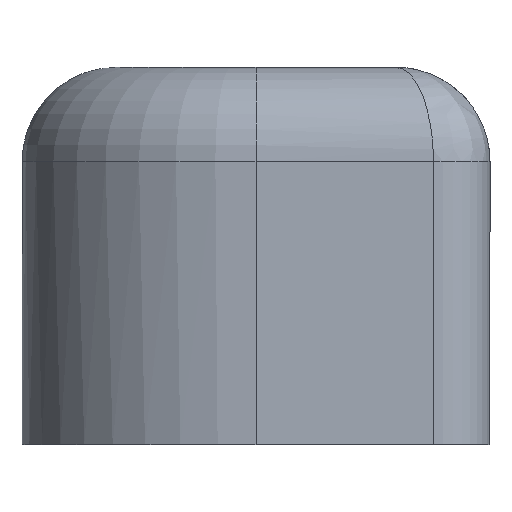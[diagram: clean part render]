
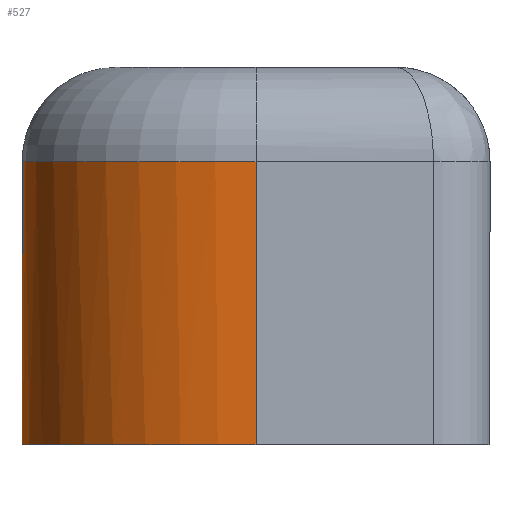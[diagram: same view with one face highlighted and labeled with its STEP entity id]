
A CAD part, left-side view. The second image highlights one B-rep face of the part: STEP entity #527.
In plain terms, the highlighted cylindrical face has radius 12.4 mm (diameter 24.8 mm), a partial arc.
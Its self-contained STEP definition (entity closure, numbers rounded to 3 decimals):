
#21 = EDGE_LOOP ( 'NONE', ( #532, #1045, #985, #869, #1587 ) ) ;
#67 = LINE ( 'NONE', #338, #1532 ) ;
#197 = FACE_OUTER_BOUND ( 'NONE', #21, .T. ) ;
#216 = DIRECTION ( 'NONE',  ( 0., 1., 0. ) ) ;
#225 = EDGE_CURVE ( 'NONE', #1175, #1431, #1409, .T. ) ;
#236 = CARTESIAN_POINT ( 'NONE',  ( -109.708, 12.4, 15. ) ) ;
#338 = CARTESIAN_POINT ( 'NONE',  ( -109.708, 12.4, -194.388 ) ) ;
#346 = DIRECTION ( 'NONE',  ( 0., 0., 1. ) ) ;
#354 = CARTESIAN_POINT ( 'NONE',  ( -97.308, 24.8, -194.388 ) ) ;
#377 = CYLINDRICAL_SURFACE ( 'NONE', #1010, 12.4 ) ;
#388 = CARTESIAN_POINT ( 'NONE',  ( -97.308, 24.8, 15. ) ) ;
#397 = CARTESIAN_POINT ( 'NONE',  ( -98.209, 24.769, 0. ) ) ;
#457 = DIRECTION ( 'NONE',  ( 0., 0., 1. ) ) ;
#458 = VERTEX_POINT ( 'NONE', #1559 ) ;
#523 = AXIS2_PLACEMENT_3D ( 'NONE', #555, #1404, #701 ) ;
#527 = ADVANCED_FACE ( 'NONE', ( #197 ), #377, .T. ) ;
#532 = ORIENTED_EDGE ( 'NONE', *, *, #225, .F. ) ;
#555 = CARTESIAN_POINT ( 'NONE',  ( -97.308, 12.4, 0. ) ) ;
#634 = CIRCLE ( 'NONE', #523, 12.4 ) ;
#639 = EDGE_CURVE ( 'NONE', #1431, #1059, #1581, .T. ) ;
#648 = VERTEX_POINT ( 'NONE', #1234 ) ;
#673 = EDGE_CURVE ( 'NONE', #458, #1059, #67, .T. ) ;
#701 = DIRECTION ( 'NONE',  ( 0., 1., 0. ) ) ;
#747 = CARTESIAN_POINT ( 'NONE',  ( -97.308, 12.4, -194.388 ) ) ;
#809 = CARTESIAN_POINT ( 'NONE',  ( -97.67, 24.796, 0.044 ) ) ;
#869 = ORIENTED_EDGE ( 'NONE', *, *, #673, .T. ) ;
#887 = B_SPLINE_CURVE_WITH_KNOTS ( 'NONE', 3,
 ( #1198, #397, #1501, #809, #1607, #955 ),
 .UNSPECIFIED., .F., .F.,
 ( 4, 2, 4 ),
 ( 0., 0.001, 0.001 ),
 .UNSPECIFIED. ) ;
#955 = CARTESIAN_POINT ( 'NONE',  ( -97.308, 24.8, 0.057 ) ) ;
#985 = ORIENTED_EDGE ( 'NONE', *, *, #1187, .T. ) ;
#1010 = AXIS2_PLACEMENT_3D ( 'NONE', #747, #1257, #1142 ) ;
#1031 = DIRECTION ( 'NONE',  ( 0., 0., 1. ) ) ;
#1045 = ORIENTED_EDGE ( 'NONE', *, *, #1457, .F. ) ;
#1059 = VERTEX_POINT ( 'NONE', #236 ) ;
#1142 = DIRECTION ( 'NONE',  ( 0., 1., 0. ) ) ;
#1175 = VERTEX_POINT ( 'NONE', #1399 ) ;
#1187 = EDGE_CURVE ( 'NONE', #648, #458, #634, .T. ) ;
#1198 = CARTESIAN_POINT ( 'NONE',  ( -98.39, 24.753, 0. ) ) ;
#1234 = CARTESIAN_POINT ( 'NONE',  ( -98.39, 24.753, 0. ) ) ;
#1244 = CARTESIAN_POINT ( 'NONE',  ( -97.308, 12.4, 15. ) ) ;
#1257 = DIRECTION ( 'NONE',  ( 0., 0., 1. ) ) ;
#1286 = VECTOR ( 'NONE', #346, 1000. ) ;
#1361 = AXIS2_PLACEMENT_3D ( 'NONE', #1244, #1031, #216 ) ;
#1399 = CARTESIAN_POINT ( 'NONE',  ( -97.308, 24.8, 0.057 ) ) ;
#1404 = DIRECTION ( 'NONE',  ( 0., 0., 1. ) ) ;
#1409 = LINE ( 'NONE', #354, #1286 ) ;
#1431 = VERTEX_POINT ( 'NONE', #388 ) ;
#1457 = EDGE_CURVE ( 'NONE', #648, #1175, #887, .T. ) ;
#1501 = CARTESIAN_POINT ( 'NONE',  ( -98.03, 24.78, 0.015 ) ) ;
#1532 = VECTOR ( 'NONE', #457, 1000. ) ;
#1559 = CARTESIAN_POINT ( 'NONE',  ( -109.708, 12.4, 0. ) ) ;
#1581 = CIRCLE ( 'NONE', #1361, 12.4 ) ;
#1587 = ORIENTED_EDGE ( 'NONE', *, *, #639, .F. ) ;
#1607 = CARTESIAN_POINT ( 'NONE',  ( -97.489, 24.8, 0.057 ) ) ;
